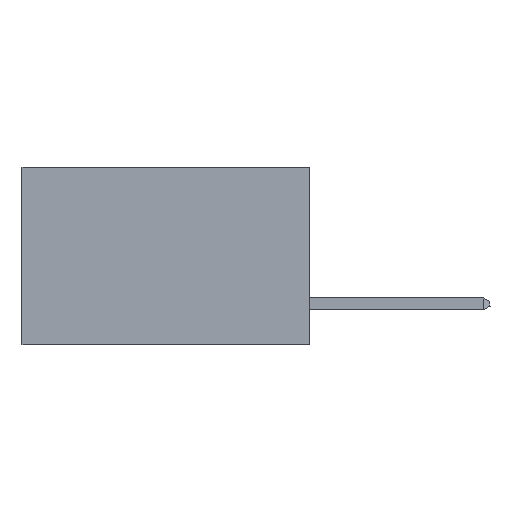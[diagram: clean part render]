
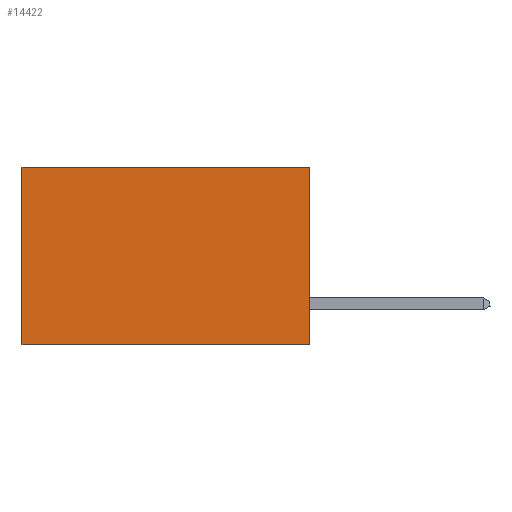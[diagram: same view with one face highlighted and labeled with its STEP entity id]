
A CAD part, left-side view. The second image highlights one B-rep face of the part: STEP entity #14422.
In plain terms, the highlighted planar face has unit normal (-1, 0, 0).
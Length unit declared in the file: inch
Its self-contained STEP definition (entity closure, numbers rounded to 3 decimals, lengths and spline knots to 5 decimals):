
#385 = VERTEX_POINT ( 'NONE', #16897 ) ;
#555 = LINE ( 'NONE', #12209, #3643 ) ;
#620 = AXIS2_PLACEMENT_3D ( 'NONE', #10529, #15941, #16129 ) ;
#2496 = EDGE_CURVE ( 'NONE', #11172, #10790, #7429, .T. ) ;
#2633 = EDGE_CURVE ( 'NONE', #10879, #385, #555, .T. ) ;
#3376 = DIRECTION ( 'NONE',  ( 0., 1., 0. ) ) ;
#3634 = ORIENTED_EDGE ( 'NONE', *, *, #12659, .F. ) ;
#3643 = VECTOR ( 'NONE', #5203, 39.37008 ) ;
#4946 = CARTESIAN_POINT ( 'NONE',  ( 0.2875, 0.6, 0. ) ) ;
#5203 = DIRECTION ( 'NONE',  ( 0., 0., -1. ) ) ;
#5709 = CARTESIAN_POINT ( 'NONE',  ( 0.2875, 0., -0.37 ) ) ;
#5970 = VECTOR ( 'NONE', #15485, 39.37008 ) ;
#6870 = CARTESIAN_POINT ( 'NONE',  ( 0.2875, 0., 0. ) ) ;
#6996 = VECTOR ( 'NONE', #17618, 39.37008 ) ;
#7364 = VECTOR ( 'NONE', #3376, 39.37008 ) ;
#7429 = LINE ( 'NONE', #9103, #6996 ) ;
#8304 = ORIENTED_EDGE ( 'NONE', *, *, #2633, .T. ) ;
#9103 = CARTESIAN_POINT ( 'NONE',  ( 0.2875, 0., 0. ) ) ;
#9731 = LINE ( 'NONE', #15213, #5970 ) ;
#10529 = CARTESIAN_POINT ( 'NONE',  ( 0.2875, 0., 0. ) ) ;
#10790 = VERTEX_POINT ( 'NONE', #5709 ) ;
#10879 = VERTEX_POINT ( 'NONE', #4946 ) ;
#11117 = LINE ( 'NONE', #6870, #7364 ) ;
#11172 = VERTEX_POINT ( 'NONE', #14118 ) ;
#11513 = EDGE_CURVE ( 'NONE', #11172, #10879, #11117, .T. ) ;
#12141 = FACE_OUTER_BOUND ( 'NONE', #13327, .T. ) ;
#12209 = CARTESIAN_POINT ( 'NONE',  ( 0.2875, 0.6, 0. ) ) ;
#12659 = EDGE_CURVE ( 'NONE', #10790, #385, #9731, .T. ) ;
#13327 = EDGE_LOOP ( 'NONE', ( #8304, #3634, #17650, #13810 ) ) ;
#13810 = ORIENTED_EDGE ( 'NONE', *, *, #11513, .T. ) ;
#14118 = CARTESIAN_POINT ( 'NONE',  ( 0.2875, 0., 0. ) ) ;
#14422 = ADVANCED_FACE ( 'NONE', ( #12141 ), #17510, .F. ) ;
#15213 = CARTESIAN_POINT ( 'NONE',  ( 0.2875, 0., -0.37 ) ) ;
#15485 = DIRECTION ( 'NONE',  ( 0., 1., 0. ) ) ;
#15941 = DIRECTION ( 'NONE',  ( 1., 0., 0. ) ) ;
#16129 = DIRECTION ( 'NONE',  ( 0., 0., -1. ) ) ;
#16897 = CARTESIAN_POINT ( 'NONE',  ( 0.2875, 0.6, -0.37 ) ) ;
#17510 = PLANE ( 'NONE',  #620 ) ;
#17618 = DIRECTION ( 'NONE',  ( 0., 0., -1. ) ) ;
#17650 = ORIENTED_EDGE ( 'NONE', *, *, #2496, .F. ) ;
